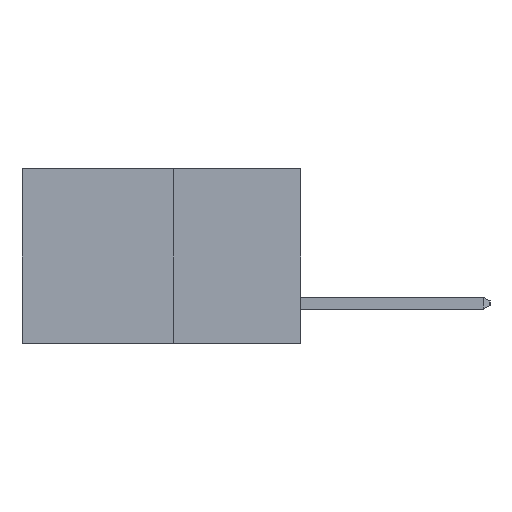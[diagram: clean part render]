
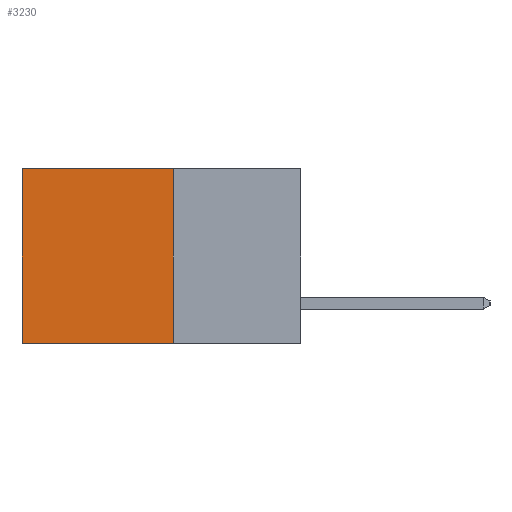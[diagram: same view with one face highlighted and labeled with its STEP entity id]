
A CAD part, left-side view. The second image highlights one B-rep face of the part: STEP entity #3230.
In plain terms, the highlighted planar face has unit normal (-1, 0, 0).
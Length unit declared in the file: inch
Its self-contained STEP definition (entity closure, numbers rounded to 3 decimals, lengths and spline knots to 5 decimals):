
#54 = EDGE_CURVE ( 'NONE', #6010, #4209, #3219, .T. ) ;
#863 = ORIENTED_EDGE ( 'NONE', *, *, #54, .T. ) ;
#965 = CARTESIAN_POINT ( 'NONE',  ( 0.277, 0.27, 0. ) ) ;
#970 = DIRECTION ( 'NONE',  ( 0., 0., -1. ) ) ;
#991 = DIRECTION ( 'NONE',  ( 0., 0., -1. ) ) ;
#1043 = CARTESIAN_POINT ( 'NONE',  ( 0.277, 0.27, -0.37 ) ) ;
#1149 = DIRECTION ( 'NONE',  ( 0., 1., 0. ) ) ;
#1933 = EDGE_CURVE ( 'NONE', #2497, #4209, #4356, .T. ) ;
#2288 = AXIS2_PLACEMENT_3D ( 'NONE', #1043, #8690, #8657 ) ;
#2311 = VECTOR ( 'NONE', #2558, 39.37008 ) ;
#2419 = ORIENTED_EDGE ( 'NONE', *, *, #2799, .F. ) ;
#2497 = VERTEX_POINT ( 'NONE', #6143 ) ;
#2558 = DIRECTION ( 'NONE',  ( 0., 1., 0. ) ) ;
#2705 = ORIENTED_EDGE ( 'NONE', *, *, #3012, .T. ) ;
#2799 = EDGE_CURVE ( 'NONE', #9590, #2497, #5409, .T. ) ;
#3012 = EDGE_CURVE ( 'NONE', #9590, #6010, #5050, .T. ) ;
#3219 = LINE ( 'NONE', #7346, #3469 ) ;
#3230 = ADVANCED_FACE ( 'NONE', ( #6922 ), #4175, .F. ) ;
#3469 = VECTOR ( 'NONE', #991, 39.37008 ) ;
#3598 = CARTESIAN_POINT ( 'NONE',  ( 0.277, 0.27, 0. ) ) ;
#3947 = EDGE_LOOP ( 'NONE', ( #863, #7064, #2419, #2705 ) ) ;
#4175 = PLANE ( 'NONE',  #2288 ) ;
#4209 = VERTEX_POINT ( 'NONE', #7795 ) ;
#4356 = LINE ( 'NONE', #4483, #2311 ) ;
#4483 = CARTESIAN_POINT ( 'NONE',  ( 0.277, 0.27, -0.37 ) ) ;
#4615 = CARTESIAN_POINT ( 'NONE',  ( 0.277, 0.27, -0.37 ) ) ;
#5050 = LINE ( 'NONE', #965, #5278 ) ;
#5278 = VECTOR ( 'NONE', #1149, 39.37008 ) ;
#5409 = LINE ( 'NONE', #4615, #5669 ) ;
#5669 = VECTOR ( 'NONE', #970, 39.37008 ) ;
#6010 = VERTEX_POINT ( 'NONE', #6784 ) ;
#6143 = CARTESIAN_POINT ( 'NONE',  ( 0.277, 0.27, -0.37 ) ) ;
#6784 = CARTESIAN_POINT ( 'NONE',  ( 0.277, 0.59, 0. ) ) ;
#6922 = FACE_OUTER_BOUND ( 'NONE', #3947, .T. ) ;
#7064 = ORIENTED_EDGE ( 'NONE', *, *, #1933, .F. ) ;
#7346 = CARTESIAN_POINT ( 'NONE',  ( 0.277, 0.59, -0.37 ) ) ;
#7795 = CARTESIAN_POINT ( 'NONE',  ( 0.277, 0.59, -0.37 ) ) ;
#8657 = DIRECTION ( 'NONE',  ( 0., 0., -1. ) ) ;
#8690 = DIRECTION ( 'NONE',  ( 1., 0., 0. ) ) ;
#9590 = VERTEX_POINT ( 'NONE', #3598 ) ;
